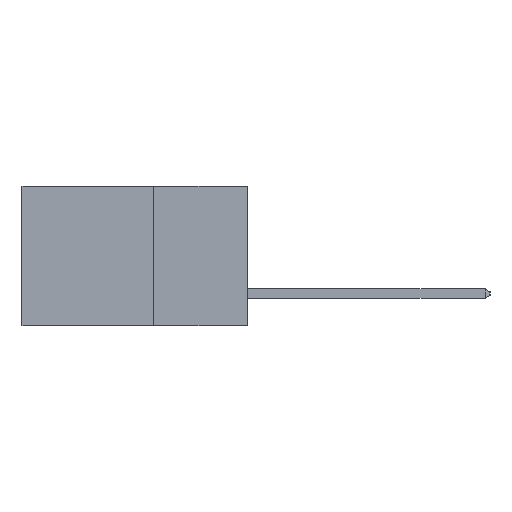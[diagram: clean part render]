
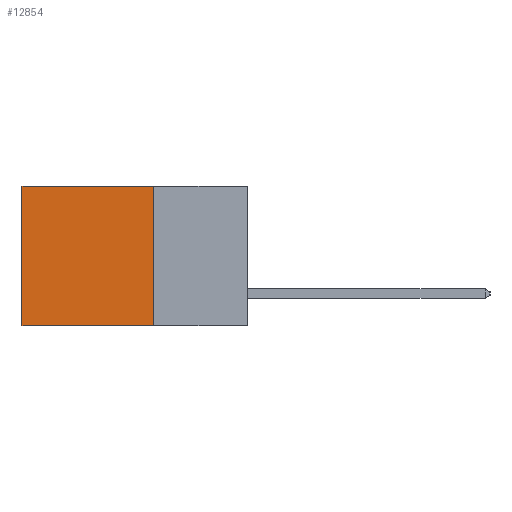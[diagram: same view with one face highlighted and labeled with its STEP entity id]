
A CAD part, left-side view. The second image highlights one B-rep face of the part: STEP entity #12854.
In plain terms, the highlighted planar face has unit normal (-1, 0, 0).
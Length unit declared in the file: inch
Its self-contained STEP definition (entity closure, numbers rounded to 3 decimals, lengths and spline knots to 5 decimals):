
#21 = VERTEX_POINT ( 'NONE', #15919 ) ;
#2048 = VECTOR ( 'NONE', #17064, 39.37008 ) ;
#3202 = ORIENTED_EDGE ( 'NONE', *, *, #13090, .T. ) ;
#4526 = DIRECTION ( 'NONE',  ( 0., 1., 0. ) ) ;
#5756 = CARTESIAN_POINT ( 'NONE',  ( 0.2615, 0.25, 0. ) ) ;
#6317 = CARTESIAN_POINT ( 'NONE',  ( 0.2615, 0.25, 0. ) ) ;
#6396 = EDGE_CURVE ( 'NONE', #7125, #11427, #6650, .T. ) ;
#6650 = LINE ( 'NONE', #16710, #2048 ) ;
#6782 = VERTEX_POINT ( 'NONE', #6317 ) ;
#7125 = VERTEX_POINT ( 'NONE', #9830 ) ;
#7612 = VECTOR ( 'NONE', #8239, 39.37008 ) ;
#8100 = VECTOR ( 'NONE', #4526, 39.37008 ) ;
#8163 = LINE ( 'NONE', #8264, #7612 ) ;
#8239 = DIRECTION ( 'NONE',  ( 0., 0., -1. ) ) ;
#8264 = CARTESIAN_POINT ( 'NONE',  ( 0.2615, 0.6, -0.37 ) ) ;
#8388 = ORIENTED_EDGE ( 'NONE', *, *, #11861, .T. ) ;
#9126 = LINE ( 'NONE', #5756, #8100 ) ;
#9380 = EDGE_CURVE ( 'NONE', #6782, #7125, #21299, .T. ) ;
#9830 = CARTESIAN_POINT ( 'NONE',  ( 0.2615, 0.25, -0.37 ) ) ;
#10143 = ORIENTED_EDGE ( 'NONE', *, *, #6396, .F. ) ;
#10809 = VECTOR ( 'NONE', #13385, 39.37008 ) ;
#11427 = VERTEX_POINT ( 'NONE', #15158 ) ;
#11861 = EDGE_CURVE ( 'NONE', #21, #11427, #8163, .T. ) ;
#12854 = ADVANCED_FACE ( 'NONE', ( #17488 ), #13418, .F. ) ;
#13066 = AXIS2_PLACEMENT_3D ( 'NONE', #14243, #13406, #13272 ) ;
#13090 = EDGE_CURVE ( 'NONE', #6782, #21, #9126, .T. ) ;
#13272 = DIRECTION ( 'NONE',  ( 0., 0., -1. ) ) ;
#13385 = DIRECTION ( 'NONE',  ( 0., 0., -1. ) ) ;
#13406 = DIRECTION ( 'NONE',  ( 1., 0., 0. ) ) ;
#13418 = PLANE ( 'NONE',  #13066 ) ;
#13602 = CARTESIAN_POINT ( 'NONE',  ( 0.2615, 0.25, -0.37 ) ) ;
#14243 = CARTESIAN_POINT ( 'NONE',  ( 0.2615, 0.25, -0.37 ) ) ;
#15158 = CARTESIAN_POINT ( 'NONE',  ( 0.2615, 0.6, -0.37 ) ) ;
#15919 = CARTESIAN_POINT ( 'NONE',  ( 0.2615, 0.6, 0. ) ) ;
#15967 = ORIENTED_EDGE ( 'NONE', *, *, #9380, .F. ) ;
#16710 = CARTESIAN_POINT ( 'NONE',  ( 0.2615, 0.25, -0.37 ) ) ;
#17064 = DIRECTION ( 'NONE',  ( 0., 1., 0. ) ) ;
#17488 = FACE_OUTER_BOUND ( 'NONE', #20407, .T. ) ;
#20407 = EDGE_LOOP ( 'NONE', ( #8388, #10143, #15967, #3202 ) ) ;
#21299 = LINE ( 'NONE', #13602, #10809 ) ;
